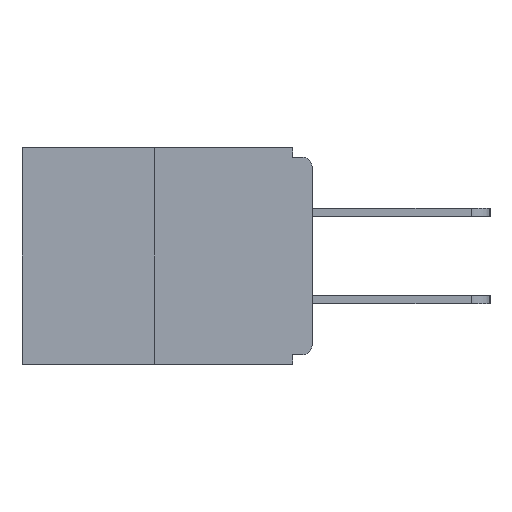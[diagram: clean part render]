
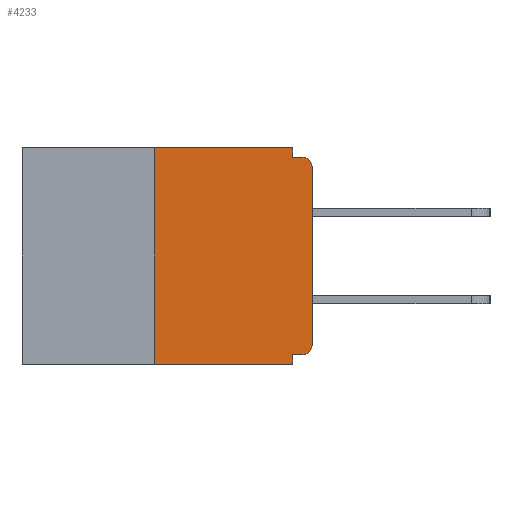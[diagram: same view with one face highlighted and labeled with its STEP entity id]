
A CAD part, left-side view. The second image highlights one B-rep face of the part: STEP entity #4233.
In plain terms, the highlighted planar face has unit normal (-1, 0, 0).
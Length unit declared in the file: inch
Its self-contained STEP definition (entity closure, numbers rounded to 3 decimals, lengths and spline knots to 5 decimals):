
#202 = VERTEX_POINT ( 'NONE', #8067 ) ;
#293 = PLANE ( 'NONE',  #11647 ) ;
#349 = ORIENTED_EDGE ( 'NONE', *, *, #12453, .F. ) ;
#548 = CARTESIAN_POINT ( 'NONE',  ( 0., 0.015, -0.313 ) ) ;
#676 = VECTOR ( 'NONE', #4481, 39.37008 ) ;
#834 = VECTOR ( 'NONE', #9047, 39.37008 ) ;
#977 = EDGE_CURVE ( 'NONE', #11488, #10017, #5161, .T. ) ;
#1616 = ORIENTED_EDGE ( 'NONE', *, *, #1647, .F. ) ;
#1647 = EDGE_CURVE ( 'NONE', #202, #14031, #3036, .T. ) ;
#2201 = CARTESIAN_POINT ( 'NONE',  ( 0., 0.25, 0. ) ) ;
#2253 = EDGE_CURVE ( 'NONE', #202, #2429, #16558, .T. ) ;
#2429 = VERTEX_POINT ( 'NONE', #6194 ) ;
#2779 = EDGE_CURVE ( 'NONE', #16697, #10017, #12177, .T. ) ;
#3036 = LINE ( 'NONE', #7291, #3504 ) ;
#3353 = CARTESIAN_POINT ( 'NONE',  ( 0., 0.46, 0. ) ) ;
#3504 = VECTOR ( 'NONE', #7415, 39.37008 ) ;
#3777 = VERTEX_POINT ( 'NONE', #12395 ) ;
#3839 = CARTESIAN_POINT ( 'NONE',  ( 0., 0.015, -0.03 ) ) ;
#4076 = ORIENTED_EDGE ( 'NONE', *, *, #977, .T. ) ;
#4233 = ADVANCED_FACE ( 'NONE', ( #10040 ), #293, .F. ) ;
#4481 = DIRECTION ( 'NONE',  ( 0., -1., 0. ) ) ;
#4696 = DIRECTION ( 'NONE',  ( 0., 0., -1. ) ) ;
#4732 = LINE ( 'NONE', #14720, #16860 ) ;
#4859 = LINE ( 'NONE', #11475, #5505 ) ;
#5161 = CIRCLE ( 'NONE', #7266, 0.015 ) ;
#5505 = VECTOR ( 'NONE', #14470, 39.37008 ) ;
#5788 = CARTESIAN_POINT ( 'NONE',  ( 0., 0., -0.015 ) ) ;
#5811 = VECTOR ( 'NONE', #12456, 39.37008 ) ;
#5815 = CARTESIAN_POINT ( 'NONE',  ( 0., 0.031, -0.328 ) ) ;
#5825 = DIRECTION ( 'NONE',  ( 0., -1., 0. ) ) ;
#6082 = DIRECTION ( 'NONE',  ( 0., 0., -1. ) ) ;
#6194 = CARTESIAN_POINT ( 'NONE',  ( 0., 0., -0.313 ) ) ;
#6396 = VECTOR ( 'NONE', #4696, 39.37008 ) ;
#6612 = DIRECTION ( 'NONE',  ( -1., 0., 0. ) ) ;
#7243 = ORIENTED_EDGE ( 'NONE', *, *, #16868, .T. ) ;
#7252 = CARTESIAN_POINT ( 'NONE',  ( 0., 0.031, 0. ) ) ;
#7266 = AXIS2_PLACEMENT_3D ( 'NONE', #3839, #6612, #16798 ) ;
#7291 = CARTESIAN_POINT ( 'NONE',  ( 0., 0., -0.328 ) ) ;
#7327 = EDGE_CURVE ( 'NONE', #2429, #11488, #4859, .T. ) ;
#7415 = DIRECTION ( 'NONE',  ( 0., 1., 0. ) ) ;
#7499 = ORIENTED_EDGE ( 'NONE', *, *, #8468, .F. ) ;
#8067 = CARTESIAN_POINT ( 'NONE',  ( 0., 0.015, -0.328 ) ) ;
#8457 = DIRECTION ( 'NONE',  ( 0., 0., 1. ) ) ;
#8468 = EDGE_CURVE ( 'NONE', #13173, #12498, #16272, .T. ) ;
#8572 = LINE ( 'NONE', #15173, #5811 ) ;
#8995 = DIRECTION ( 'NONE',  ( 1., 0., 0. ) ) ;
#8996 = VECTOR ( 'NONE', #8457, 39.37008 ) ;
#9047 = DIRECTION ( 'NONE',  ( 0., -1., 0. ) ) ;
#9267 = ORIENTED_EDGE ( 'NONE', *, *, #7327, .T. ) ;
#9438 = DIRECTION ( 'NONE',  ( -1., 0., 0. ) ) ;
#9542 = CARTESIAN_POINT ( 'NONE',  ( 0., 0.015, -0.015 ) ) ;
#9927 = CARTESIAN_POINT ( 'NONE',  ( 0., 0.25, 0. ) ) ;
#10017 = VERTEX_POINT ( 'NONE', #9542 ) ;
#10040 = FACE_OUTER_BOUND ( 'NONE', #10768, .T. ) ;
#10768 = EDGE_LOOP ( 'NONE', ( #7499, #349, #7243, #14154, #1616, #15573, #9267, #4076, #14776, #16896 ) ) ;
#11280 = CARTESIAN_POINT ( 'NONE',  ( 0., 0.031, 0. ) ) ;
#11460 = AXIS2_PLACEMENT_3D ( 'NONE', #548, #9438, #13820 ) ;
#11475 = CARTESIAN_POINT ( 'NONE',  ( 0., 0., 0. ) ) ;
#11488 = VERTEX_POINT ( 'NONE', #17627 ) ;
#11647 = AXIS2_PLACEMENT_3D ( 'NONE', #15062, #8995, #6082 ) ;
#11683 = CARTESIAN_POINT ( 'NONE',  ( 0., 0.031, -0.343 ) ) ;
#12177 = LINE ( 'NONE', #5788, #676 ) ;
#12395 = CARTESIAN_POINT ( 'NONE',  ( 0., 0.25, -0.343 ) ) ;
#12453 = EDGE_CURVE ( 'NONE', #3777, #13173, #18609, .T. ) ;
#12456 = DIRECTION ( 'NONE',  ( 0., 0., -1. ) ) ;
#12498 = VERTEX_POINT ( 'NONE', #11280 ) ;
#13173 = VERTEX_POINT ( 'NONE', #2201 ) ;
#13308 = EDGE_CURVE ( 'NONE', #12498, #16697, #14503, .T. ) ;
#13820 = DIRECTION ( 'NONE',  ( 0., 0., -1. ) ) ;
#14031 = VERTEX_POINT ( 'NONE', #5815 ) ;
#14154 = ORIENTED_EDGE ( 'NONE', *, *, #18286, .F. ) ;
#14470 = DIRECTION ( 'NONE',  ( 0., 0., 1. ) ) ;
#14503 = LINE ( 'NONE', #7252, #6396 ) ;
#14720 = CARTESIAN_POINT ( 'NONE',  ( 0., 0.46, -0.343 ) ) ;
#14776 = ORIENTED_EDGE ( 'NONE', *, *, #2779, .F. ) ;
#15062 = CARTESIAN_POINT ( 'NONE',  ( 0., 0.46, 0. ) ) ;
#15173 = CARTESIAN_POINT ( 'NONE',  ( 0., 0.031, -0.343 ) ) ;
#15573 = ORIENTED_EDGE ( 'NONE', *, *, #2253, .T. ) ;
#16272 = LINE ( 'NONE', #3353, #834 ) ;
#16281 = VERTEX_POINT ( 'NONE', #11683 ) ;
#16558 = CIRCLE ( 'NONE', #11460, 0.015 ) ;
#16697 = VERTEX_POINT ( 'NONE', #16768 ) ;
#16768 = CARTESIAN_POINT ( 'NONE',  ( 0., 0.031, -0.015 ) ) ;
#16798 = DIRECTION ( 'NONE',  ( 0., 0., -1. ) ) ;
#16860 = VECTOR ( 'NONE', #5825, 39.37008 ) ;
#16868 = EDGE_CURVE ( 'NONE', #3777, #16281, #4732, .T. ) ;
#16896 = ORIENTED_EDGE ( 'NONE', *, *, #13308, .F. ) ;
#17627 = CARTESIAN_POINT ( 'NONE',  ( 0., 0., -0.03 ) ) ;
#18286 = EDGE_CURVE ( 'NONE', #14031, #16281, #8572, .T. ) ;
#18609 = LINE ( 'NONE', #9927, #8996 ) ;
